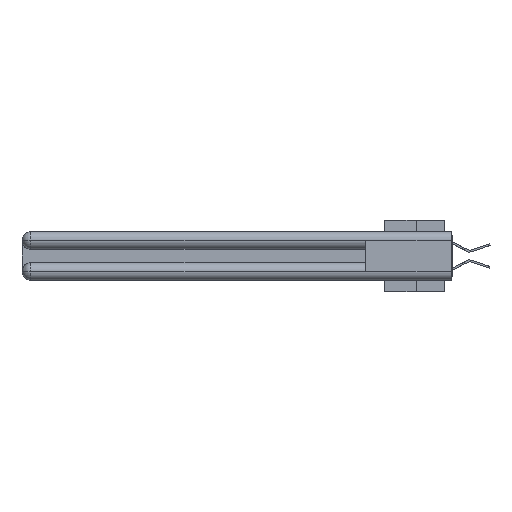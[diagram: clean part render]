
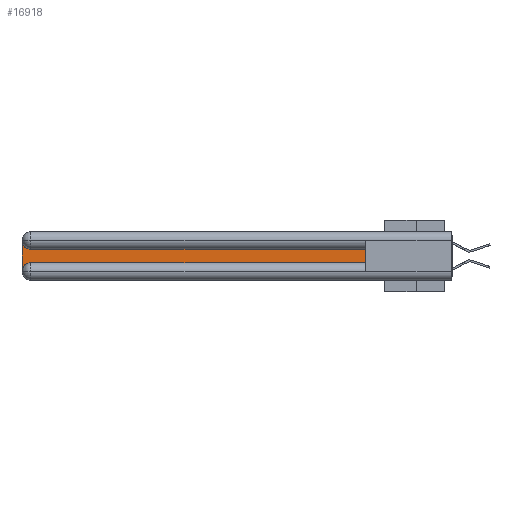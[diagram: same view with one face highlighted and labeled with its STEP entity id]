
A CAD part, left-side view. The second image highlights one B-rep face of the part: STEP entity #16918.
In plain terms, the highlighted planar face has unit normal (-1, 0, 0).
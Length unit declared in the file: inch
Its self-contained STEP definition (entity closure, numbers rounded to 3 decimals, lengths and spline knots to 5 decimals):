
#728 = LINE ( 'NONE', #15636, #6794 ) ;
#1005 = DIRECTION ( 'NONE',  ( 0., 1., 0. ) ) ;
#1806 = DIRECTION ( 'NONE',  ( 1., 0., 0. ) ) ;
#1864 = VERTEX_POINT ( 'NONE', #16455 ) ;
#2526 = CARTESIAN_POINT ( 'NONE',  ( 0.075, 3., -0.2775 ) ) ;
#3461 = ORIENTED_EDGE ( 'NONE', *, *, #24117, .T. ) ;
#4020 = ORIENTED_EDGE ( 'NONE', *, *, #14214, .T. ) ;
#4146 = CARTESIAN_POINT ( 'NONE',  ( 0.075, 3., -0.2175 ) ) ;
#4245 = DIRECTION ( 'NONE',  ( 0., 0., -1. ) ) ;
#4269 = CARTESIAN_POINT ( 'NONE',  ( 0.075, 0.6, -0.1225 ) ) ;
#4584 = EDGE_CURVE ( 'NONE', #14633, #17873, #728, .T. ) ;
#4623 = AXIS2_PLACEMENT_3D ( 'NONE', #11443, #1806, #4245 ) ;
#5011 = DIRECTION ( 'NONE',  ( 0., 0., 1. ) ) ;
#5289 = CARTESIAN_POINT ( 'NONE',  ( 0.075, 2.94, -0.1225 ) ) ;
#6031 = LINE ( 'NONE', #9420, #24591 ) ;
#6794 = VECTOR ( 'NONE', #1005, 39.37008 ) ;
#7530 = CIRCLE ( 'NONE', #4623, 0.06 ) ;
#7892 = CARTESIAN_POINT ( 'NONE',  ( 0.075, 0.6, -0.2175 ) ) ;
#7993 = LINE ( 'NONE', #4146, #25805 ) ;
#9134 = CARTESIAN_POINT ( 'NONE',  ( 0.075, 2.94, -0.0625 ) ) ;
#9420 = CARTESIAN_POINT ( 'NONE',  ( 0.075, 0.6, -0.2175 ) ) ;
#10446 = PLANE ( 'NONE',  #16568 ) ;
#11232 = FACE_OUTER_BOUND ( 'NONE', #13640, .T. ) ;
#11443 = CARTESIAN_POINT ( 'NONE',  ( 0.075, 2.94, -0.2775 ) ) ;
#12139 = VECTOR ( 'NONE', #17434, 39.37008 ) ;
#13229 = CIRCLE ( 'NONE', #24514, 0.06 ) ;
#13640 = EDGE_LOOP ( 'NONE', ( #27226, #3461, #18910, #16132, #18849, #4020 ) ) ;
#13833 = DIRECTION ( 'NONE',  ( 1., 0., 0. ) ) ;
#14214 = EDGE_CURVE ( 'NONE', #1864, #14633, #6031, .T. ) ;
#14633 = VERTEX_POINT ( 'NONE', #4269 ) ;
#15636 = CARTESIAN_POINT ( 'NONE',  ( 0.075, 0.6, -0.1225 ) ) ;
#16132 = ORIENTED_EDGE ( 'NONE', *, *, #23489, .T. ) ;
#16455 = CARTESIAN_POINT ( 'NONE',  ( 0.075, 0.6, -0.2175 ) ) ;
#16568 = AXIS2_PLACEMENT_3D ( 'NONE', #27815, #30041, #18000 ) ;
#16918 = ADVANCED_FACE ( 'NONE', ( #11232 ), #10446, .F. ) ;
#17434 = DIRECTION ( 'NONE',  ( 0., -1., 0. ) ) ;
#17873 = VERTEX_POINT ( 'NONE', #5289 ) ;
#18000 = DIRECTION ( 'NONE',  ( 0., 0., -1. ) ) ;
#18849 = ORIENTED_EDGE ( 'NONE', *, *, #30774, .T. ) ;
#18910 = ORIENTED_EDGE ( 'NONE', *, *, #22700, .T. ) ;
#22700 = EDGE_CURVE ( 'NONE', #31091, #30630, #7993, .T. ) ;
#23489 = EDGE_CURVE ( 'NONE', #30630, #28358, #7530, .T. ) ;
#23663 = CARTESIAN_POINT ( 'NONE',  ( 0.075, 2.94, -0.2175 ) ) ;
#24117 = EDGE_CURVE ( 'NONE', #17873, #31091, #13229, .T. ) ;
#24514 = AXIS2_PLACEMENT_3D ( 'NONE', #9134, #13833, #26074 ) ;
#24591 = VECTOR ( 'NONE', #5011, 39.37008 ) ;
#25805 = VECTOR ( 'NONE', #28453, 39.37008 ) ;
#26074 = DIRECTION ( 'NONE',  ( 0., 0., -1. ) ) ;
#27226 = ORIENTED_EDGE ( 'NONE', *, *, #4584, .T. ) ;
#27815 = CARTESIAN_POINT ( 'NONE',  ( 0.075, 3., -0.1225 ) ) ;
#28358 = VERTEX_POINT ( 'NONE', #23663 ) ;
#28453 = DIRECTION ( 'NONE',  ( 0., 0., -1. ) ) ;
#30041 = DIRECTION ( 'NONE',  ( 1., 0., 0. ) ) ;
#30269 = LINE ( 'NONE', #7892, #12139 ) ;
#30625 = CARTESIAN_POINT ( 'NONE',  ( 0.075, 3., -0.0625 ) ) ;
#30630 = VERTEX_POINT ( 'NONE', #2526 ) ;
#30774 = EDGE_CURVE ( 'NONE', #28358, #1864, #30269, .T. ) ;
#31091 = VERTEX_POINT ( 'NONE', #30625 ) ;
